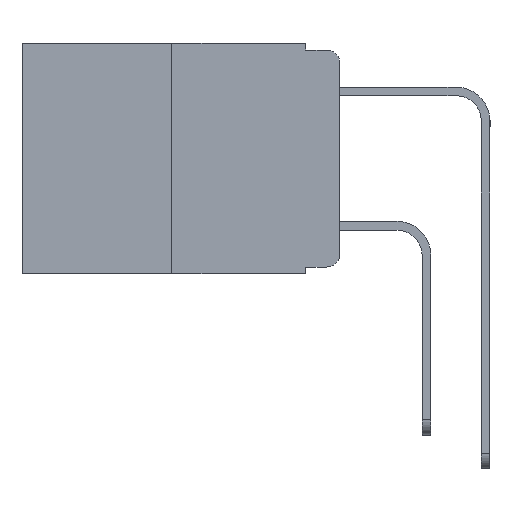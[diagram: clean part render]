
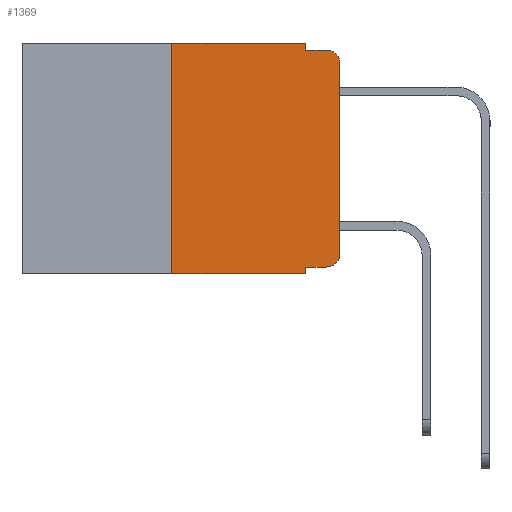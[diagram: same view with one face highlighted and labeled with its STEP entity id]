
A CAD part, left-side view. The second image highlights one B-rep face of the part: STEP entity #1369.
In plain terms, the highlighted planar face has unit normal (-1, 0, 0).
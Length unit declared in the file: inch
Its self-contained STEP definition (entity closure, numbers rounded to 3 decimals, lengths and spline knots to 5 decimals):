
#228 = VERTEX_POINT ( 'NONE', #17594 ) ;
#247 = EDGE_CURVE ( 'NONE', #5230, #292, #1389, .T. ) ;
#288 = LINE ( 'NONE', #15590, #17611 ) ;
#292 = VERTEX_POINT ( 'NONE', #7807 ) ;
#349 = ORIENTED_EDGE ( 'NONE', *, *, #5108, .T. ) ;
#373 = DIRECTION ( 'NONE',  ( -1., 0., 0. ) ) ;
#495 = ORIENTED_EDGE ( 'NONE', *, *, #11931, .T. ) ;
#571 = VERTEX_POINT ( 'NONE', #19581 ) ;
#1306 = ORIENTED_EDGE ( 'NONE', *, *, #2760, .F. ) ;
#1369 = ADVANCED_FACE ( 'NONE', ( #12620 ), #10792, .F. ) ;
#1389 = LINE ( 'NONE', #20117, #5559 ) ;
#1518 = EDGE_CURVE ( 'NONE', #19278, #19830, #5780, .T. ) ;
#1544 = CARTESIAN_POINT ( 'NONE',  ( 0., 0.051, 0. ) ) ;
#1586 = CARTESIAN_POINT ( 'NONE',  ( 0., 0.051, 0. ) ) ;
#1639 = VECTOR ( 'NONE', #11442, 39.37008 ) ;
#1739 = ORIENTED_EDGE ( 'NONE', *, *, #18604, .F. ) ;
#2044 = CARTESIAN_POINT ( 'NONE',  ( 0., 0., -0.313 ) ) ;
#2151 = ORIENTED_EDGE ( 'NONE', *, *, #247, .F. ) ;
#2266 = CARTESIAN_POINT ( 'NONE',  ( 0., 0.02, -0.333 ) ) ;
#2553 = CARTESIAN_POINT ( 'NONE',  ( 0., 0.051, -0.343 ) ) ;
#2760 = EDGE_CURVE ( 'NONE', #19830, #571, #5186, .T. ) ;
#3448 = EDGE_LOOP ( 'NONE', ( #15884, #349, #1306, #13090, #4321, #2151, #495, #1739, #6434, #9057 ) ) ;
#4073 = CARTESIAN_POINT ( 'NONE',  ( 0., 0.051, -0.333 ) ) ;
#4256 = CARTESIAN_POINT ( 'NONE',  ( 0., 0.051, -0.01 ) ) ;
#4321 = ORIENTED_EDGE ( 'NONE', *, *, #14259, .F. ) ;
#5108 = EDGE_CURVE ( 'NONE', #7401, #571, #7336, .T. ) ;
#5186 = LINE ( 'NONE', #4256, #12300 ) ;
#5230 = VERTEX_POINT ( 'NONE', #8792 ) ;
#5559 = VECTOR ( 'NONE', #10423, 39.37008 ) ;
#5780 = LINE ( 'NONE', #1544, #9021 ) ;
#5781 = DIRECTION ( 'NONE',  ( 0., -1., 0. ) ) ;
#5791 = LINE ( 'NONE', #9774, #1639 ) ;
#5918 = DIRECTION ( 'NONE',  ( 0., -1., 0. ) ) ;
#5953 = DIRECTION ( 'NONE',  ( 0., -1., 0. ) ) ;
#6070 = VERTEX_POINT ( 'NONE', #2266 ) ;
#6222 = EDGE_CURVE ( 'NONE', #13080, #7401, #13688, .T. ) ;
#6434 = ORIENTED_EDGE ( 'NONE', *, *, #16472, .T. ) ;
#6524 = CARTESIAN_POINT ( 'NONE',  ( 0., 0.051, -0.01 ) ) ;
#6994 = CARTESIAN_POINT ( 'NONE',  ( 0., 0.02, -0.03 ) ) ;
#7336 = CIRCLE ( 'NONE', #12644, 0.02 ) ;
#7401 = VERTEX_POINT ( 'NONE', #17264 ) ;
#7438 = VECTOR ( 'NONE', #19195, 39.37008 ) ;
#7564 = DIRECTION ( 'NONE',  ( 0., 0., -1. ) ) ;
#7807 = CARTESIAN_POINT ( 'NONE',  ( 0., 0.25, 0. ) ) ;
#8582 = DIRECTION ( 'NONE',  ( 0., 0., -1. ) ) ;
#8792 = CARTESIAN_POINT ( 'NONE',  ( 0., 0.25, -0.343 ) ) ;
#8806 = VECTOR ( 'NONE', #12629, 39.37008 ) ;
#8991 = AXIS2_PLACEMENT_3D ( 'NONE', #12870, #11180, #21069 ) ;
#9021 = VECTOR ( 'NONE', #7564, 39.37008 ) ;
#9057 = ORIENTED_EDGE ( 'NONE', *, *, #13138, .T. ) ;
#9774 = CARTESIAN_POINT ( 'NONE',  ( 0., 0.473, 0. ) ) ;
#10423 = DIRECTION ( 'NONE',  ( 0., 0., 1. ) ) ;
#10575 = CARTESIAN_POINT ( 'NONE',  ( 0., 0.02, -0.313 ) ) ;
#10782 = LINE ( 'NONE', #4073, #19438 ) ;
#10792 = PLANE ( 'NONE',  #8991 ) ;
#10985 = CARTESIAN_POINT ( 'NONE',  ( 0., 0., 0. ) ) ;
#11180 = DIRECTION ( 'NONE',  ( 1., 0., 0. ) ) ;
#11442 = DIRECTION ( 'NONE',  ( 0., -1., 0. ) ) ;
#11922 = CIRCLE ( 'NONE', #17935, 0.02 ) ;
#11931 = EDGE_CURVE ( 'NONE', #5230, #15272, #288, .T. ) ;
#12231 = DIRECTION ( 'NONE',  ( 0., 0., -1. ) ) ;
#12300 = VECTOR ( 'NONE', #5953, 39.37008 ) ;
#12620 = FACE_OUTER_BOUND ( 'NONE', #3448, .T. ) ;
#12629 = DIRECTION ( 'NONE',  ( 0., 0., 1. ) ) ;
#12644 = AXIS2_PLACEMENT_3D ( 'NONE', #6994, #18376, #8582 ) ;
#12870 = CARTESIAN_POINT ( 'NONE',  ( 0., 0.473, 0. ) ) ;
#13080 = VERTEX_POINT ( 'NONE', #2044 ) ;
#13090 = ORIENTED_EDGE ( 'NONE', *, *, #1518, .F. ) ;
#13138 = EDGE_CURVE ( 'NONE', #6070, #13080, #11922, .T. ) ;
#13688 = LINE ( 'NONE', #10985, #8806 ) ;
#14259 = EDGE_CURVE ( 'NONE', #292, #19278, #5791, .T. ) ;
#15272 = VERTEX_POINT ( 'NONE', #2553 ) ;
#15590 = CARTESIAN_POINT ( 'NONE',  ( 0., 0.473, -0.343 ) ) ;
#15884 = ORIENTED_EDGE ( 'NONE', *, *, #6222, .T. ) ;
#16133 = LINE ( 'NONE', #17672, #7438 ) ;
#16472 = EDGE_CURVE ( 'NONE', #228, #6070, #10782, .T. ) ;
#17264 = CARTESIAN_POINT ( 'NONE',  ( 0., 0., -0.03 ) ) ;
#17594 = CARTESIAN_POINT ( 'NONE',  ( 0., 0.051, -0.333 ) ) ;
#17611 = VECTOR ( 'NONE', #5918, 39.37008 ) ;
#17672 = CARTESIAN_POINT ( 'NONE',  ( 0., 0.051, 0. ) ) ;
#17935 = AXIS2_PLACEMENT_3D ( 'NONE', #10575, #373, #12231 ) ;
#18376 = DIRECTION ( 'NONE',  ( -1., 0., 0. ) ) ;
#18604 = EDGE_CURVE ( 'NONE', #228, #15272, #16133, .T. ) ;
#19195 = DIRECTION ( 'NONE',  ( 0., 0., -1. ) ) ;
#19278 = VERTEX_POINT ( 'NONE', #1586 ) ;
#19438 = VECTOR ( 'NONE', #5781, 39.37008 ) ;
#19581 = CARTESIAN_POINT ( 'NONE',  ( 0., 0.02, -0.01 ) ) ;
#19830 = VERTEX_POINT ( 'NONE', #6524 ) ;
#20117 = CARTESIAN_POINT ( 'NONE',  ( 0., 0.25, 0. ) ) ;
#21069 = DIRECTION ( 'NONE',  ( 0., 0., -1. ) ) ;
